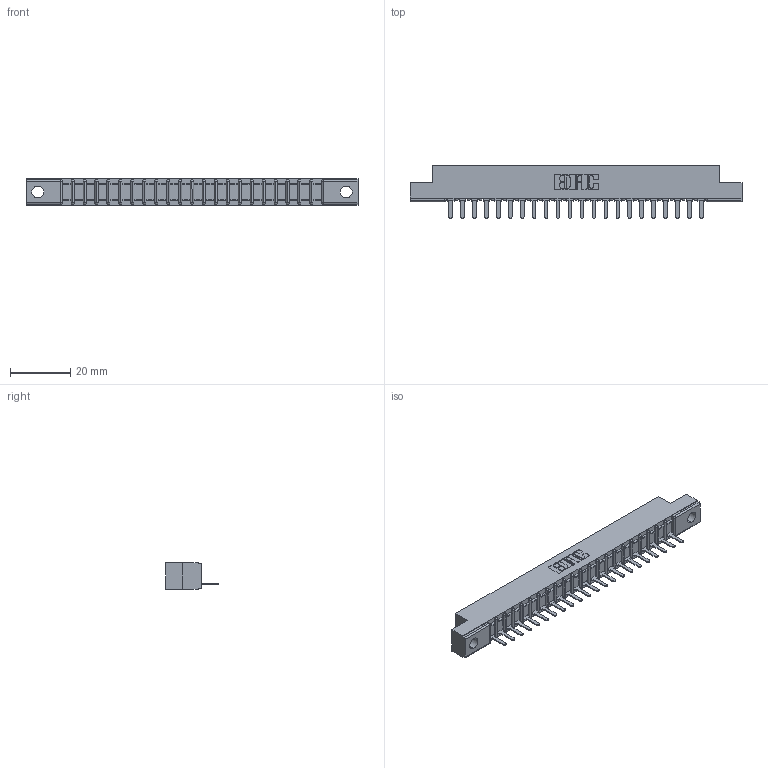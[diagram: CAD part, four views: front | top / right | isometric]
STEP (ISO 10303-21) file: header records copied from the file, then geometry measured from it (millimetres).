
FILE_DESCRIPTION (( 'STEP AP203' ), '1' );
FILE_NAME ('307-022-521-104.STEP', '2018-08-04T03:39:43', ( '' ), ( '' ), 'SwSTEP 2.0', 'SolidWorks 2016', '' );
FILE_SCHEMA (( 'CONFIG_CONTROL_DESIGN' ));
Length unit declared in the file: inch
Products named in the file (3): 307 Part_.156 Dia Mounting Holes; 307-290-002_521; 307-022-521-104
Assembly tree (23 placements, depth 2):
  307-022-521-104
    307 Part_.156 Dia Mounting Holes
    307-290-002_521  x22
Bounding box: 110.19 x 17.42 x 8.71 mm (x, y, z)
Volume: 7169.6 mm3; surface area: 12944.2 mm2
Topology: 23 solids, 23 shells, 1783 faces, 5463 edges, 3578 vertices
Faces by surface type: plane 1074, cylinder 663, sphere 46
Entity records: 22462 total; most frequent: CARTESIAN_POINT 3790, ORIENTED_EDGE 3778, DIRECTION 3683, EDGE_CURVE 1889, LINE 1445, VECTOR 1445, VERTEX_POINT 1226, AXIS2_PLACEMENT_3D 1119
